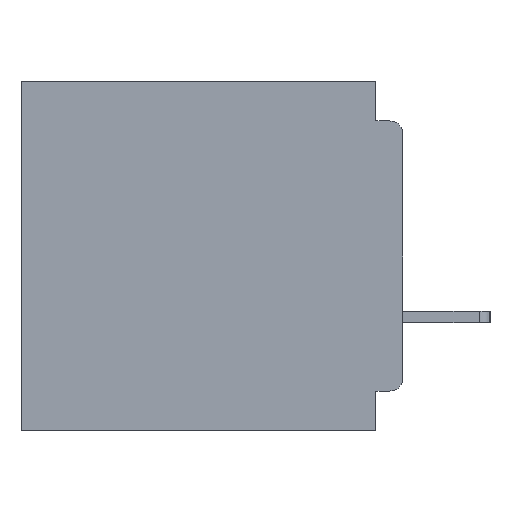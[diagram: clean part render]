
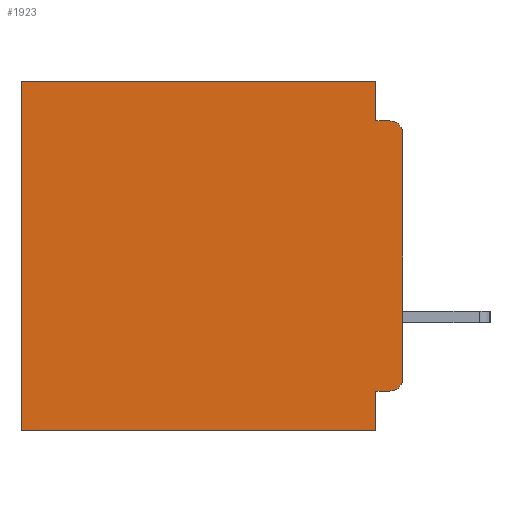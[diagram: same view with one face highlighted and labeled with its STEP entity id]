
A CAD part, left-side view. The second image highlights one B-rep face of the part: STEP entity #1923.
In plain terms, the highlighted planar face has unit normal (-1, 0, 0).
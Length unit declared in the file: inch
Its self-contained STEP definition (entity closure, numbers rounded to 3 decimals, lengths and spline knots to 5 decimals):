
#274 = CARTESIAN_POINT ( 'NONE',  ( 0.3, 0., -0.34 ) ) ;
#1223 = LINE ( 'NONE', #1460, #12497 ) ;
#1460 = CARTESIAN_POINT ( 'NONE',  ( 0.3, 0., -0.4 ) ) ;
#1575 = CARTESIAN_POINT ( 'NONE',  ( 0.3, 0.015, -0.34 ) ) ;
#1850 = CARTESIAN_POINT ( 'NONE',  ( 0.3, 0.437, 0. ) ) ;
#1923 = ADVANCED_FACE ( 'NONE', ( #48527 ), #53413, .F. ) ;
#1926 = CARTESIAN_POINT ( 'NONE',  ( 0.3, 0.031, 0. ) ) ;
#2331 = DIRECTION ( 'NONE',  ( 0., 0., -1. ) ) ;
#2820 = VECTOR ( 'NONE', #35458, 39.37008 ) ;
#3289 = VERTEX_POINT ( 'NONE', #19685 ) ;
#4306 = VERTEX_POINT ( 'NONE', #1850 ) ;
#4674 = CARTESIAN_POINT ( 'NONE',  ( 0.3, 0., -0.06 ) ) ;
#5038 = CIRCLE ( 'NONE', #54076, 0.015 ) ;
#5844 = DIRECTION ( 'NONE',  ( 0., 0., -1. ) ) ;
#9442 = VERTEX_POINT ( 'NONE', #29145 ) ;
#9601 = VECTOR ( 'NONE', #48387, 39.37008 ) ;
#10608 = ORIENTED_EDGE ( 'NONE', *, *, #43601, .T. ) ;
#10796 = CARTESIAN_POINT ( 'NONE',  ( 0.3, 0.015, -0.355 ) ) ;
#11907 = LINE ( 'NONE', #45075, #32985 ) ;
#12497 = VECTOR ( 'NONE', #43384, 39.37008 ) ;
#12991 = VERTEX_POINT ( 'NONE', #38801 ) ;
#14457 = EDGE_CURVE ( 'NONE', #50289, #20700, #49077, .T. ) ;
#16015 = LINE ( 'NONE', #45629, #38348 ) ;
#17588 = CARTESIAN_POINT ( 'NONE',  ( 0.3, 0., -0.4 ) ) ;
#17723 = VERTEX_POINT ( 'NONE', #45357 ) ;
#17761 = CARTESIAN_POINT ( 'NONE',  ( 0.3, 0.031, -0.4 ) ) ;
#18805 = EDGE_CURVE ( 'NONE', #37652, #17723, #11907, .T. ) ;
#19085 = CARTESIAN_POINT ( 'NONE',  ( 0.3, 0., 0. ) ) ;
#19685 = CARTESIAN_POINT ( 'NONE',  ( 0.3, 0.031, 0. ) ) ;
#20700 = VERTEX_POINT ( 'NONE', #25404 ) ;
#20819 = LINE ( 'NONE', #19085, #9601 ) ;
#20846 = EDGE_CURVE ( 'NONE', #17723, #12991, #51786, .T. ) ;
#20973 = LINE ( 'NONE', #17588, #44554 ) ;
#22396 = LINE ( 'NONE', #1926, #33541 ) ;
#23857 = DIRECTION ( 'NONE',  ( -1., 0., 0. ) ) ;
#24636 = VERTEX_POINT ( 'NONE', #47315 ) ;
#24652 = ORIENTED_EDGE ( 'NONE', *, *, #18805, .F. ) ;
#24853 = DIRECTION ( 'NONE',  ( 0., -1., 0. ) ) ;
#25404 = CARTESIAN_POINT ( 'NONE',  ( 0.3, 0.015, -0.045 ) ) ;
#27859 = ORIENTED_EDGE ( 'NONE', *, *, #51635, .T. ) ;
#29145 = CARTESIAN_POINT ( 'NONE',  ( 0.3, 0.437, -0.4 ) ) ;
#30102 = EDGE_CURVE ( 'NONE', #12991, #9442, #1223, .T. ) ;
#31090 = ORIENTED_EDGE ( 'NONE', *, *, #14457, .T. ) ;
#31101 = DIRECTION ( 'NONE',  ( -1., 0., 0. ) ) ;
#31253 = CARTESIAN_POINT ( 'NONE',  ( 0.3, 0.437, -0.4 ) ) ;
#31469 = DIRECTION ( 'NONE',  ( 0., 0., -1. ) ) ;
#32985 = VECTOR ( 'NONE', #36710, 39.37008 ) ;
#33541 = VECTOR ( 'NONE', #31469, 39.37008 ) ;
#34701 = DIRECTION ( 'NONE',  ( 0., 0., -1. ) ) ;
#35458 = DIRECTION ( 'NONE',  ( 0., 0., -1. ) ) ;
#35666 = AXIS2_PLACEMENT_3D ( 'NONE', #48879, #23857, #52992 ) ;
#36442 = LINE ( 'NONE', #31253, #2820 ) ;
#36687 = ORIENTED_EDGE ( 'NONE', *, *, #50301, .F. ) ;
#36710 = DIRECTION ( 'NONE',  ( 0., 1., 0. ) ) ;
#36740 = VERTEX_POINT ( 'NONE', #274 ) ;
#37652 = VERTEX_POINT ( 'NONE', #10796 ) ;
#38348 = VECTOR ( 'NONE', #24853, 39.37008 ) ;
#38801 = CARTESIAN_POINT ( 'NONE',  ( 0.3, 0.031, -0.4 ) ) ;
#40728 = VECTOR ( 'NONE', #34701, 39.37008 ) ;
#40758 = EDGE_LOOP ( 'NONE', ( #36687, #31090, #53586, #47648, #10608, #45745, #52058, #46870, #24652, #27859 ) ) ;
#43384 = DIRECTION ( 'NONE',  ( 0., 1., 0. ) ) ;
#43601 = EDGE_CURVE ( 'NONE', #3289, #4306, #20819, .T. ) ;
#44554 = VECTOR ( 'NONE', #46919, 39.37008 ) ;
#45075 = CARTESIAN_POINT ( 'NONE',  ( 0.3, 0., -0.355 ) ) ;
#45357 = CARTESIAN_POINT ( 'NONE',  ( 0.3, 0.031, -0.355 ) ) ;
#45629 = CARTESIAN_POINT ( 'NONE',  ( 0.3, 0., -0.045 ) ) ;
#45745 = ORIENTED_EDGE ( 'NONE', *, *, #53521, .T. ) ;
#46870 = ORIENTED_EDGE ( 'NONE', *, *, #20846, .F. ) ;
#46919 = DIRECTION ( 'NONE',  ( 0., 0., -1. ) ) ;
#47315 = CARTESIAN_POINT ( 'NONE',  ( 0.3, 0.031, -0.045 ) ) ;
#47648 = ORIENTED_EDGE ( 'NONE', *, *, #49853, .F. ) ;
#48387 = DIRECTION ( 'NONE',  ( 0., 1., 0. ) ) ;
#48527 = FACE_OUTER_BOUND ( 'NONE', #40758, .T. ) ;
#48879 = CARTESIAN_POINT ( 'NONE',  ( 0.3, 0.015, -0.06 ) ) ;
#49077 = CIRCLE ( 'NONE', #35666, 0.015 ) ;
#49853 = EDGE_CURVE ( 'NONE', #3289, #24636, #22396, .T. ) ;
#50289 = VERTEX_POINT ( 'NONE', #4674 ) ;
#50301 = EDGE_CURVE ( 'NONE', #50289, #36740, #20973, .T. ) ;
#51240 = AXIS2_PLACEMENT_3D ( 'NONE', #52699, #51401, #2331 ) ;
#51401 = DIRECTION ( 'NONE',  ( 1., 0., 0. ) ) ;
#51635 = EDGE_CURVE ( 'NONE', #37652, #36740, #5038, .T. ) ;
#51786 = LINE ( 'NONE', #17761, #40728 ) ;
#52058 = ORIENTED_EDGE ( 'NONE', *, *, #30102, .F. ) ;
#52699 = CARTESIAN_POINT ( 'NONE',  ( 0.3, 0., -0.4 ) ) ;
#52992 = DIRECTION ( 'NONE',  ( 0., 0., -1. ) ) ;
#53413 = PLANE ( 'NONE',  #51240 ) ;
#53521 = EDGE_CURVE ( 'NONE', #4306, #9442, #36442, .T. ) ;
#53586 = ORIENTED_EDGE ( 'NONE', *, *, #53709, .F. ) ;
#53709 = EDGE_CURVE ( 'NONE', #24636, #20700, #16015, .T. ) ;
#54076 = AXIS2_PLACEMENT_3D ( 'NONE', #1575, #31101, #5844 ) ;
